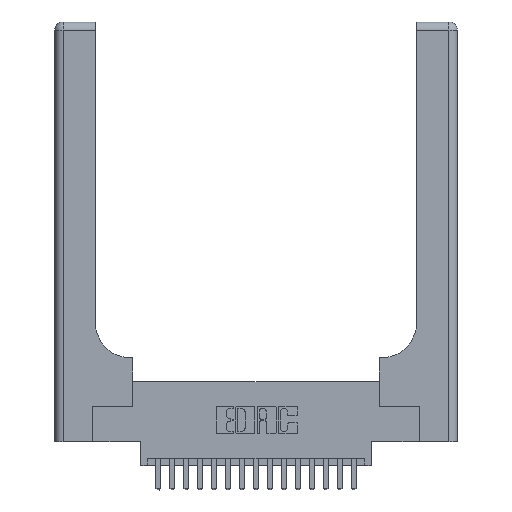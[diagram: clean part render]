
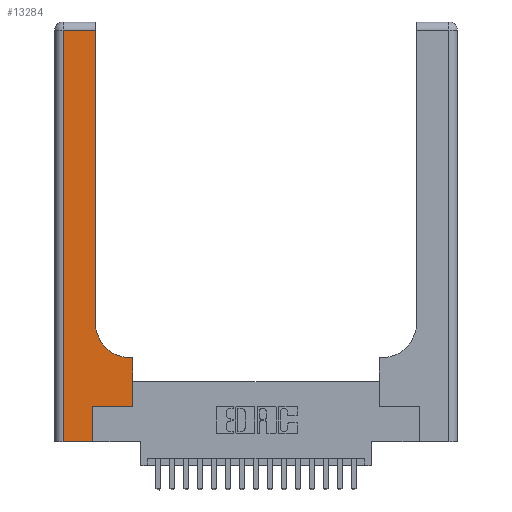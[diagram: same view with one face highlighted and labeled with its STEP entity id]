
A CAD part, top view. The second image highlights one B-rep face of the part: STEP entity #13284.
In plain terms, the highlighted planar face has unit normal (0, 0, 1).
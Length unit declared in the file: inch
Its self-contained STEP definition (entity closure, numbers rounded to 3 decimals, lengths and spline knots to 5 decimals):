
#759 = VECTOR ( 'NONE', #17023, 39.37008 ) ;
#772 = CARTESIAN_POINT ( 'NONE',  ( 0., 2.94, 0.37 ) ) ;
#1023 = VERTEX_POINT ( 'NONE', #5023 ) ;
#1084 = VERTEX_POINT ( 'NONE', #13998 ) ;
#1301 = DIRECTION ( 'NONE',  ( 1., 0., 0. ) ) ;
#2282 = LINE ( 'NONE', #4033, #20126 ) ;
#2557 = CARTESIAN_POINT ( 'NONE',  ( 0.2915, 0.85, 0.37 ) ) ;
#2594 = ORIENTED_EDGE ( 'NONE', *, *, #19978, .T. ) ;
#2661 = DIRECTION ( 'NONE',  ( 0., -1., 0. ) ) ;
#3752 = AXIS2_PLACEMENT_3D ( 'NONE', #5258, #7086, #16806 ) ;
#4009 = LINE ( 'NONE', #12700, #5752 ) ;
#4033 = CARTESIAN_POINT ( 'NONE',  ( 0.269, 0., 0.37 ) ) ;
#4557 = EDGE_CURVE ( 'NONE', #1084, #4766, #2282, .T. ) ;
#4733 = EDGE_CURVE ( 'NONE', #1023, #16251, #19400, .T. ) ;
#4766 = VERTEX_POINT ( 'NONE', #7998 ) ;
#5013 = CARTESIAN_POINT ( 'NONE',  ( 0.5585, 0.25, 0.37 ) ) ;
#5023 = CARTESIAN_POINT ( 'NONE',  ( 0.5415, 0.6, 0.37 ) ) ;
#5258 = CARTESIAN_POINT ( 'NONE',  ( 0.5415, 0.85, 0.37 ) ) ;
#5310 = DIRECTION ( 'NONE',  ( 0., 1., 0. ) ) ;
#5448 = EDGE_LOOP ( 'NONE', ( #20804, #18365, #17132, #16116, #10470, #13328, #11253, #2594, #14170 ) ) ;
#5533 = LINE ( 'NONE', #772, #759 ) ;
#5752 = VECTOR ( 'NONE', #12835, 39.37008 ) ;
#5810 = CARTESIAN_POINT ( 'NONE',  ( 0.06, 0., 0.37 ) ) ;
#7086 = DIRECTION ( 'NONE',  ( 0., 0., -1. ) ) ;
#7684 = VECTOR ( 'NONE', #10530, 39.37008 ) ;
#7998 = CARTESIAN_POINT ( 'NONE',  ( 0.269, 0.25, 0.37 ) ) ;
#8436 = VECTOR ( 'NONE', #2661, 39.37008 ) ;
#8471 = CARTESIAN_POINT ( 'NONE',  ( 0.5585, 0.25, 0.37 ) ) ;
#8475 = LINE ( 'NONE', #15728, #16530 ) ;
#8622 = CARTESIAN_POINT ( 'NONE',  ( 0.06, 2.94, 0.37 ) ) ;
#8663 = LINE ( 'NONE', #8471, #11930 ) ;
#8921 = CARTESIAN_POINT ( 'NONE',  ( 0.2915, 0.6, 0.37 ) ) ;
#9169 = CARTESIAN_POINT ( 'NONE',  ( 0.2915, 3., 0.37 ) ) ;
#9941 = DIRECTION ( 'NONE',  ( 0., 1., 0. ) ) ;
#10341 = EDGE_CURVE ( 'NONE', #20249, #12321, #5533, .T. ) ;
#10470 = ORIENTED_EDGE ( 'NONE', *, *, #4557, .T. ) ;
#10530 = DIRECTION ( 'NONE',  ( -1., 0., 0. ) ) ;
#10773 = VERTEX_POINT ( 'NONE', #15371 ) ;
#11175 = VERTEX_POINT ( 'NONE', #5013 ) ;
#11253 = ORIENTED_EDGE ( 'NONE', *, *, #16561, .T. ) ;
#11261 = DIRECTION ( 'NONE',  ( 0., 0., -1. ) ) ;
#11427 = LINE ( 'NONE', #20449, #8436 ) ;
#11930 = VECTOR ( 'NONE', #9941, 39.37008 ) ;
#12321 = VERTEX_POINT ( 'NONE', #8622 ) ;
#12644 = EDGE_CURVE ( 'NONE', #4766, #11175, #4009, .T. ) ;
#12700 = CARTESIAN_POINT ( 'NONE',  ( 0.269, 0.25, 0.37 ) ) ;
#12835 = DIRECTION ( 'NONE',  ( 1., 0., 0. ) ) ;
#13284 = ADVANCED_FACE ( 'NONE', ( #19843 ), #14299, .F. ) ;
#13328 = ORIENTED_EDGE ( 'NONE', *, *, #12644, .T. ) ;
#13949 = VECTOR ( 'NONE', #13959, 39.37008 ) ;
#13959 = DIRECTION ( 'NONE',  ( 0., 1., 0. ) ) ;
#13998 = CARTESIAN_POINT ( 'NONE',  ( 0.269, 0., 0.37 ) ) ;
#14170 = ORIENTED_EDGE ( 'NONE', *, *, #4733, .T. ) ;
#14299 = PLANE ( 'NONE',  #18424 ) ;
#14320 = VERTEX_POINT ( 'NONE', #5810 ) ;
#14732 = LINE ( 'NONE', #8921, #7684 ) ;
#14773 = CARTESIAN_POINT ( 'NONE',  ( 0.2915, 2.94, 0.37 ) ) ;
#15371 = CARTESIAN_POINT ( 'NONE',  ( 0.5585, 0.6, 0.37 ) ) ;
#15711 = EDGE_CURVE ( 'NONE', #16251, #20249, #18244, .T. ) ;
#15728 = CARTESIAN_POINT ( 'NONE',  ( 0., 0., 0.37 ) ) ;
#16073 = DIRECTION ( 'NONE',  ( -1., 0., 0. ) ) ;
#16116 = ORIENTED_EDGE ( 'NONE', *, *, #19361, .T. ) ;
#16251 = VERTEX_POINT ( 'NONE', #2557 ) ;
#16530 = VECTOR ( 'NONE', #1301, 39.37008 ) ;
#16561 = EDGE_CURVE ( 'NONE', #11175, #10773, #8663, .T. ) ;
#16806 = DIRECTION ( 'NONE',  ( 1., 0., 0. ) ) ;
#17023 = DIRECTION ( 'NONE',  ( -1., 0., 0. ) ) ;
#17132 = ORIENTED_EDGE ( 'NONE', *, *, #20360, .T. ) ;
#18244 = LINE ( 'NONE', #9169, #13949 ) ;
#18365 = ORIENTED_EDGE ( 'NONE', *, *, #10341, .T. ) ;
#18424 = AXIS2_PLACEMENT_3D ( 'NONE', #19228, #11261, #16073 ) ;
#19228 = CARTESIAN_POINT ( 'NONE',  ( 0., 3., 0.37 ) ) ;
#19361 = EDGE_CURVE ( 'NONE', #14320, #1084, #8475, .T. ) ;
#19400 = CIRCLE ( 'NONE', #3752, 0.25 ) ;
#19843 = FACE_OUTER_BOUND ( 'NONE', #5448, .T. ) ;
#19978 = EDGE_CURVE ( 'NONE', #10773, #1023, #14732, .T. ) ;
#20126 = VECTOR ( 'NONE', #5310, 39.37008 ) ;
#20249 = VERTEX_POINT ( 'NONE', #14773 ) ;
#20360 = EDGE_CURVE ( 'NONE', #12321, #14320, #11427, .T. ) ;
#20449 = CARTESIAN_POINT ( 'NONE',  ( 0.06, 3., 0.37 ) ) ;
#20804 = ORIENTED_EDGE ( 'NONE', *, *, #15711, .T. ) ;
